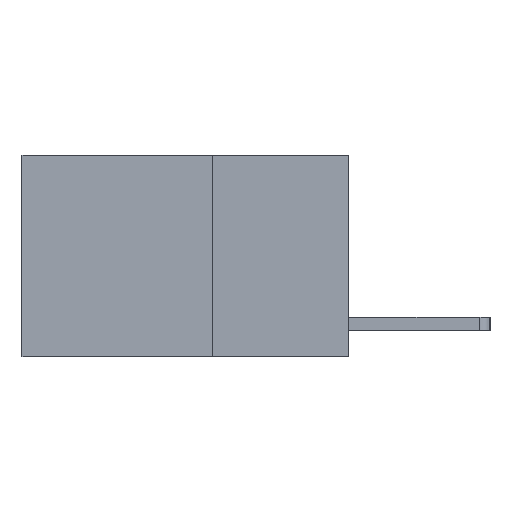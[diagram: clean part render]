
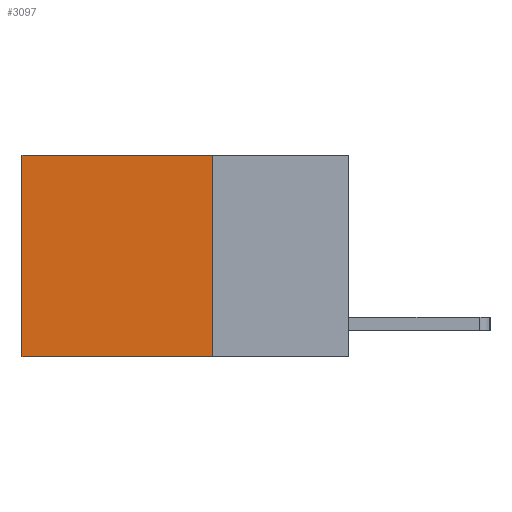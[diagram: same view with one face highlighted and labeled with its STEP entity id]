
A CAD part, left-side view. The second image highlights one B-rep face of the part: STEP entity #3097.
In plain terms, the highlighted planar face has unit normal (-1, 0, 0).
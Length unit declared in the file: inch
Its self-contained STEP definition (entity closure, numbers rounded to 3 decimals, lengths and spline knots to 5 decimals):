
#18 = CARTESIAN_POINT ( 'NONE',  ( 0.2625, 0.25, -0.37 ) ) ;
#376 = CARTESIAN_POINT ( 'NONE',  ( 0.2625, 0.25, -0.37 ) ) ;
#492 = VERTEX_POINT ( 'NONE', #10713 ) ;
#678 = EDGE_CURVE ( 'NONE', #492, #1482, #9925, .T. ) ;
#744 = DIRECTION ( 'NONE',  ( 0., 0., -1. ) ) ;
#802 = DIRECTION ( 'NONE',  ( 0., 0., -1. ) ) ;
#1273 = ORIENTED_EDGE ( 'NONE', *, *, #11037, .F. ) ;
#1482 = VERTEX_POINT ( 'NONE', #376 ) ;
#2126 = CARTESIAN_POINT ( 'NONE',  ( 0.2625, 0.6, -0.37 ) ) ;
#2361 = ORIENTED_EDGE ( 'NONE', *, *, #678, .F. ) ;
#2435 = DIRECTION ( 'NONE',  ( 0., 0., -1. ) ) ;
#2541 = EDGE_CURVE ( 'NONE', #7213, #5063, #7258, .T. ) ;
#2775 = VECTOR ( 'NONE', #802, 39.37008 ) ;
#3037 = VECTOR ( 'NONE', #3655, 39.37008 ) ;
#3097 = ADVANCED_FACE ( 'NONE', ( #8482 ), #4212, .F. ) ;
#3655 = DIRECTION ( 'NONE',  ( 0., 1., 0. ) ) ;
#4212 = PLANE ( 'NONE',  #9689 ) ;
#4473 = CARTESIAN_POINT ( 'NONE',  ( 0.2625, 0.25, 0. ) ) ;
#4842 = VECTOR ( 'NONE', #744, 39.37008 ) ;
#5063 = VERTEX_POINT ( 'NONE', #2126 ) ;
#5103 = CARTESIAN_POINT ( 'NONE',  ( 0.2625, 0.25, 0. ) ) ;
#5417 = LINE ( 'NONE', #18, #3037 ) ;
#6116 = EDGE_CURVE ( 'NONE', #492, #7213, #11285, .T. ) ;
#6433 = ORIENTED_EDGE ( 'NONE', *, *, #2541, .T. ) ;
#6769 = EDGE_LOOP ( 'NONE', ( #6433, #1273, #2361, #6896 ) ) ;
#6896 = ORIENTED_EDGE ( 'NONE', *, *, #6116, .T. ) ;
#7213 = VERTEX_POINT ( 'NONE', #9810 ) ;
#7258 = LINE ( 'NONE', #10624, #4842 ) ;
#7836 = DIRECTION ( 'NONE',  ( 1., 0., 0. ) ) ;
#8482 = FACE_OUTER_BOUND ( 'NONE', #6769, .T. ) ;
#9002 = CARTESIAN_POINT ( 'NONE',  ( 0.2625, 0.25, 0. ) ) ;
#9689 = AXIS2_PLACEMENT_3D ( 'NONE', #5103, #7836, #2435 ) ;
#9810 = CARTESIAN_POINT ( 'NONE',  ( 0.2625, 0.6, 0. ) ) ;
#9925 = LINE ( 'NONE', #9002, #2775 ) ;
#10624 = CARTESIAN_POINT ( 'NONE',  ( 0.2625, 0.6, 0. ) ) ;
#10713 = CARTESIAN_POINT ( 'NONE',  ( 0.2625, 0.25, 0. ) ) ;
#10715 = DIRECTION ( 'NONE',  ( 0., 1., 0. ) ) ;
#10994 = VECTOR ( 'NONE', #10715, 39.37008 ) ;
#11037 = EDGE_CURVE ( 'NONE', #1482, #5063, #5417, .T. ) ;
#11285 = LINE ( 'NONE', #4473, #10994 ) ;
